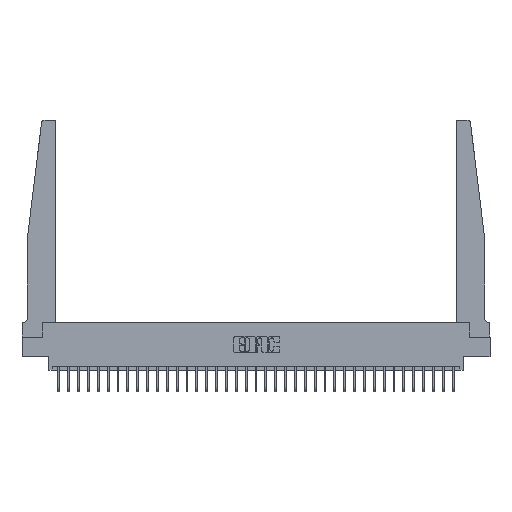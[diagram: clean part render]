
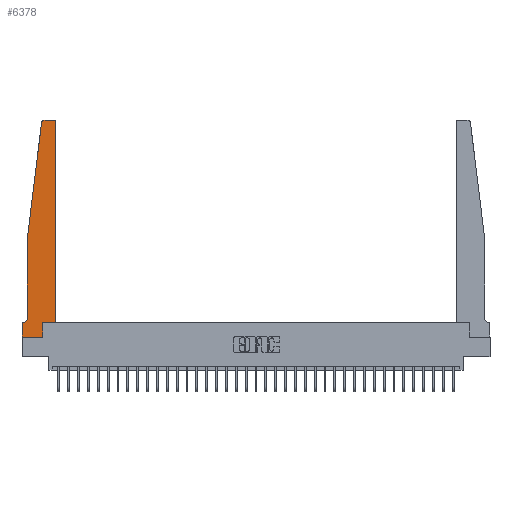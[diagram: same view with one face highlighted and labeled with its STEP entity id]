
A CAD part, top view. The second image highlights one B-rep face of the part: STEP entity #6378.
In plain terms, the highlighted planar face has unit normal (0, 0, 1).
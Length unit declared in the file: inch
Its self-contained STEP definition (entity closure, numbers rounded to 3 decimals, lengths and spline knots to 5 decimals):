
#190 = CARTESIAN_POINT ( 'NONE',  ( 0., 0., 0.37 ) ) ;
#830 = DIRECTION ( 'NONE',  ( 1., 0., 0. ) ) ;
#1052 = EDGE_CURVE ( 'NONE', #17993, #20831, #15502, .T. ) ;
#1658 = CARTESIAN_POINT ( 'NONE',  ( 0.27653, 2.72, 0.37 ) ) ;
#1932 = AXIS2_PLACEMENT_3D ( 'NONE', #9665, #10016, #22755 ) ;
#2152 = EDGE_CURVE ( 'NONE', #20831, #9989, #28093, .T. ) ;
#2276 = FACE_OUTER_BOUND ( 'NONE', #5243, .T. ) ;
#2499 = CARTESIAN_POINT ( 'NONE',  ( 0.425, 0.18, 0.37 ) ) ;
#2597 = DIRECTION ( 'NONE',  ( 0., -1., 0. ) ) ;
#2602 = ORIENTED_EDGE ( 'NONE', *, *, #29344, .T. ) ;
#3529 = VERTEX_POINT ( 'NONE', #32065 ) ;
#3644 = VECTOR ( 'NONE', #7325, 39.37008 ) ;
#3815 = LINE ( 'NONE', #19489, #33411 ) ;
#4443 = CARTESIAN_POINT ( 'NONE',  ( 0.395, 2.75, 0.37 ) ) ;
#4654 = EDGE_CURVE ( 'NONE', #5568, #3529, #31051, .T. ) ;
#5243 = EDGE_LOOP ( 'NONE', ( #32819, #20731, #26564, #10198, #11769, #14563, #32401, #2602, #15398, #8376, #26633, #5304 ) ) ;
#5304 = ORIENTED_EDGE ( 'NONE', *, *, #32063, .T. ) ;
#5324 = VECTOR ( 'NONE', #25485, 39.37008 ) ;
#5568 = VERTEX_POINT ( 'NONE', #4443 ) ;
#5823 = LINE ( 'NONE', #32004, #16089 ) ;
#6098 = CARTESIAN_POINT ( 'NONE',  ( 0.24675, 2.72367, 0.37 ) ) ;
#6378 = ADVANCED_FACE ( 'NONE', ( #2276 ), #20008, .T. ) ;
#7319 = DIRECTION ( 'NONE',  ( 0., 0., 1. ) ) ;
#7325 = DIRECTION ( 'NONE',  ( -0.122, -0.992, 0. ) ) ;
#7555 = CARTESIAN_POINT ( 'NONE',  ( 0.425, 0.18, 0.37 ) ) ;
#7764 = DIRECTION ( 'NONE',  ( -1., 0., 0. ) ) ;
#7966 = EDGE_CURVE ( 'NONE', #34007, #17570, #23230, .T. ) ;
#8376 = ORIENTED_EDGE ( 'NONE', *, *, #32799, .T. ) ;
#9070 = VERTEX_POINT ( 'NONE', #6098 ) ;
#9112 = VERTEX_POINT ( 'NONE', #13850 ) ;
#9665 = CARTESIAN_POINT ( 'NONE',  ( 0., 0.1875, 0.37 ) ) ;
#9989 = VERTEX_POINT ( 'NONE', #20472 ) ;
#10016 = DIRECTION ( 'NONE',  ( 0., 0., 1. ) ) ;
#10198 = ORIENTED_EDGE ( 'NONE', *, *, #1052, .T. ) ;
#10750 = LINE ( 'NONE', #26591, #15032 ) ;
#11375 = VECTOR ( 'NONE', #25525, 39.37008 ) ;
#11633 = CARTESIAN_POINT ( 'NONE',  ( 0.065, 1.25, 0.37 ) ) ;
#11769 = ORIENTED_EDGE ( 'NONE', *, *, #2152, .T. ) ;
#12403 = EDGE_CURVE ( 'NONE', #9989, #22086, #19692, .T. ) ;
#13238 = AXIS2_PLACEMENT_3D ( 'NONE', #31881, #29307, #7764 ) ;
#13760 = VECTOR ( 'NONE', #2597, 39.37008 ) ;
#13850 = CARTESIAN_POINT ( 'NONE',  ( 0.2605, 0., 0.37 ) ) ;
#14008 = DIRECTION ( 'NONE',  ( 1., 0., 0. ) ) ;
#14563 = ORIENTED_EDGE ( 'NONE', *, *, #12403, .T. ) ;
#15032 = VECTOR ( 'NONE', #14008, 39.37008 ) ;
#15157 = LINE ( 'NONE', #190, #13760 ) ;
#15398 = ORIENTED_EDGE ( 'NONE', *, *, #22659, .T. ) ;
#15434 = CARTESIAN_POINT ( 'NONE',  ( 0., 0.1875, 0.37 ) ) ;
#15502 = LINE ( 'NONE', #26006, #29388 ) ;
#16089 = VECTOR ( 'NONE', #830, 39.37008 ) ;
#16179 = CARTESIAN_POINT ( 'NONE',  ( 0.395, 2.72, 0.37 ) ) ;
#16673 = CIRCLE ( 'NONE', #17209, 0.03 ) ;
#17209 = AXIS2_PLACEMENT_3D ( 'NONE', #16179, #26662, #24070 ) ;
#17570 = VERTEX_POINT ( 'NONE', #32338 ) ;
#17993 = VERTEX_POINT ( 'NONE', #11633 ) ;
#19489 = CARTESIAN_POINT ( 'NONE',  ( 0.2605, 0.18, 0.37 ) ) ;
#19692 = LINE ( 'NONE', #22603, #20806 ) ;
#20008 = PLANE ( 'NONE',  #1932 ) ;
#20472 = CARTESIAN_POINT ( 'NONE',  ( 0.015, 0.1875, 0.37 ) ) ;
#20731 = ORIENTED_EDGE ( 'NONE', *, *, #22997, .T. ) ;
#20774 = EDGE_CURVE ( 'NONE', #9070, #17993, #33866, .T. ) ;
#20806 = VECTOR ( 'NONE', #30377, 39.37008 ) ;
#20831 = VERTEX_POINT ( 'NONE', #21773 ) ;
#21773 = CARTESIAN_POINT ( 'NONE',  ( 0.065, 0.2375, 0.37 ) ) ;
#22086 = VERTEX_POINT ( 'NONE', #15434 ) ;
#22603 = CARTESIAN_POINT ( 'NONE',  ( 0.065, 0.1875, 0.37 ) ) ;
#22659 = EDGE_CURVE ( 'NONE', #9112, #31126, #3815, .T. ) ;
#22755 = DIRECTION ( 'NONE',  ( 1., 0., 0. ) ) ;
#22851 = VERTEX_POINT ( 'NONE', #26299 ) ;
#22997 = EDGE_CURVE ( 'NONE', #3529, #9070, #27951, .T. ) ;
#23230 = LINE ( 'NONE', #7555, #5324 ) ;
#24070 = DIRECTION ( 'NONE',  ( 1., 0., 0. ) ) ;
#25485 = DIRECTION ( 'NONE',  ( 0., 1., 0. ) ) ;
#25525 = DIRECTION ( 'NONE',  ( -1., 0., 0. ) ) ;
#25861 = CARTESIAN_POINT ( 'NONE',  ( 0.25, 2.75, 0.37 ) ) ;
#26006 = CARTESIAN_POINT ( 'NONE',  ( 0.065, 1.25, 0.37 ) ) ;
#26299 = CARTESIAN_POINT ( 'NONE',  ( 0., 0., 0.37 ) ) ;
#26564 = ORIENTED_EDGE ( 'NONE', *, *, #20774, .T. ) ;
#26591 = CARTESIAN_POINT ( 'NONE',  ( 0.425, 0.18, 0.37 ) ) ;
#26633 = ORIENTED_EDGE ( 'NONE', *, *, #7966, .T. ) ;
#26662 = DIRECTION ( 'NONE',  ( 0., 0., 1. ) ) ;
#27139 = CARTESIAN_POINT ( 'NONE',  ( 0.2605, 0.18, 0.37 ) ) ;
#27354 = EDGE_CURVE ( 'NONE', #22086, #22851, #15157, .T. ) ;
#27951 = CIRCLE ( 'NONE', #29039, 0.03 ) ;
#28093 = CIRCLE ( 'NONE', #13238, 0.05 ) ;
#28765 = DIRECTION ( 'NONE',  ( 0., -1., 0. ) ) ;
#29039 = AXIS2_PLACEMENT_3D ( 'NONE', #1658, #7319, #30753 ) ;
#29307 = DIRECTION ( 'NONE',  ( 0., 0., -1. ) ) ;
#29344 = EDGE_CURVE ( 'NONE', #22851, #9112, #5823, .T. ) ;
#29388 = VECTOR ( 'NONE', #28765, 39.37008 ) ;
#30377 = DIRECTION ( 'NONE',  ( -1., 0., 0. ) ) ;
#30753 = DIRECTION ( 'NONE',  ( 1., 0., 0. ) ) ;
#30944 = CARTESIAN_POINT ( 'NONE',  ( 0.065, 1.25, 0.37 ) ) ;
#31051 = LINE ( 'NONE', #25861, #11375 ) ;
#31126 = VERTEX_POINT ( 'NONE', #27139 ) ;
#31881 = CARTESIAN_POINT ( 'NONE',  ( 0.015, 0.2375, 0.37 ) ) ;
#32004 = CARTESIAN_POINT ( 'NONE',  ( 0., 0., 0.37 ) ) ;
#32063 = EDGE_CURVE ( 'NONE', #17570, #5568, #16673, .T. ) ;
#32065 = CARTESIAN_POINT ( 'NONE',  ( 0.27653, 2.75, 0.37 ) ) ;
#32338 = CARTESIAN_POINT ( 'NONE',  ( 0.425, 2.72, 0.37 ) ) ;
#32401 = ORIENTED_EDGE ( 'NONE', *, *, #27354, .T. ) ;
#32799 = EDGE_CURVE ( 'NONE', #31126, #34007, #10750, .T. ) ;
#32819 = ORIENTED_EDGE ( 'NONE', *, *, #4654, .T. ) ;
#33087 = DIRECTION ( 'NONE',  ( 0., 1., 0. ) ) ;
#33411 = VECTOR ( 'NONE', #33087, 39.37008 ) ;
#33866 = LINE ( 'NONE', #30944, #3644 ) ;
#34007 = VERTEX_POINT ( 'NONE', #2499 ) ;
